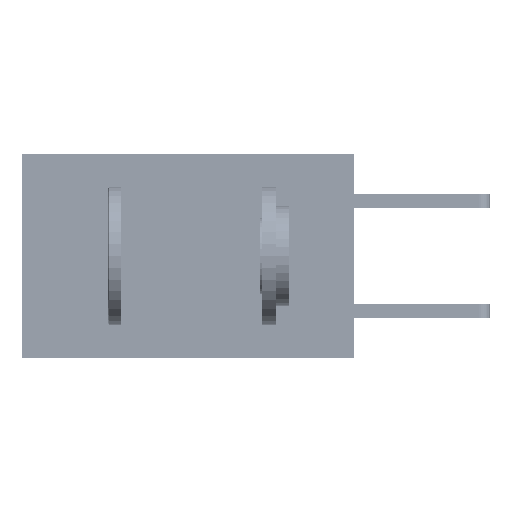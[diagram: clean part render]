
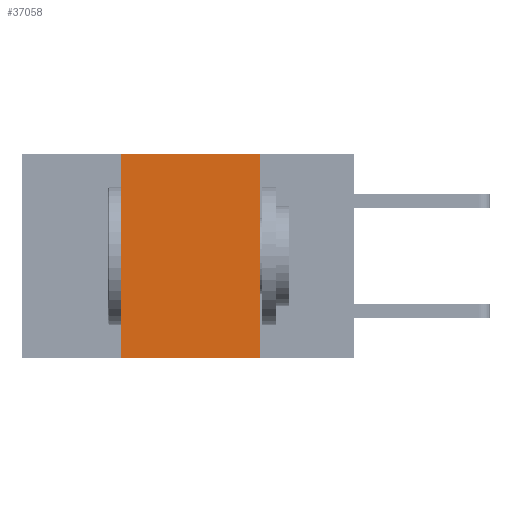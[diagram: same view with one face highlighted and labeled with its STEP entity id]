
A CAD part, left-side view. The second image highlights one B-rep face of the part: STEP entity #37058.
In plain terms, the highlighted planar face has unit normal (-1, 0, 0).
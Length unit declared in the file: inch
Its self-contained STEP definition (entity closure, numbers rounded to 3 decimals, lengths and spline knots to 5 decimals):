
#285 = EDGE_CURVE ( 'NONE', #36489, #21820, #44807, .T. ) ;
#646 = DIRECTION ( 'NONE',  ( 0., -1., 0. ) ) ;
#5187 = ORIENTED_EDGE ( 'NONE', *, *, #48113, .F. ) ;
#6625 = LINE ( 'NONE', #11080, #50487 ) ;
#7666 = VECTOR ( 'NONE', #37270, 39.37008 ) ;
#9012 = ORIENTED_EDGE ( 'NONE', *, *, #38375, .F. ) ;
#9309 = CARTESIAN_POINT ( 'NONE',  ( 0., 0.6, -0.37 ) ) ;
#9411 = CARTESIAN_POINT ( 'NONE',  ( 0., 0.17, 0. ) ) ;
#9585 = VERTEX_POINT ( 'NONE', #37923 ) ;
#9885 = CARTESIAN_POINT ( 'NONE',  ( 0., 0.17, -0.37 ) ) ;
#10435 = DIRECTION ( 'NONE',  ( 0., 0., -1. ) ) ;
#10575 = DIRECTION ( 'NONE',  ( 0., 0., 1. ) ) ;
#11080 = CARTESIAN_POINT ( 'NONE',  ( 0., 0.42, 0. ) ) ;
#11533 = VECTOR ( 'NONE', #646, 39.37008 ) ;
#13605 = DIRECTION ( 'NONE',  ( 1., 0., 0. ) ) ;
#13886 = LINE ( 'NONE', #46690, #35745 ) ;
#21116 = EDGE_CURVE ( 'NONE', #24123, #21820, #49351, .T. ) ;
#21753 = DIRECTION ( 'NONE',  ( 0., -1., 0. ) ) ;
#21820 = VERTEX_POINT ( 'NONE', #9885 ) ;
#24123 = VERTEX_POINT ( 'NONE', #9411 ) ;
#29151 = CARTESIAN_POINT ( 'NONE',  ( 0., 0.17, 0. ) ) ;
#33556 = PLANE ( 'NONE',  #47368 ) ;
#33822 = FACE_OUTER_BOUND ( 'NONE', #51465, .T. ) ;
#35745 = VECTOR ( 'NONE', #21753, 39.37008 ) ;
#36489 = VERTEX_POINT ( 'NONE', #36987 ) ;
#36987 = CARTESIAN_POINT ( 'NONE',  ( 0., 0.42, -0.37 ) ) ;
#37058 = ADVANCED_FACE ( 'NONE', ( #33822 ), #33556, .F. ) ;
#37270 = DIRECTION ( 'NONE',  ( 0., 0., -1. ) ) ;
#37923 = CARTESIAN_POINT ( 'NONE',  ( 0., 0.42, 0. ) ) ;
#38375 = EDGE_CURVE ( 'NONE', #9585, #24123, #13886, .T. ) ;
#38711 = ORIENTED_EDGE ( 'NONE', *, *, #21116, .F. ) ;
#38746 = ORIENTED_EDGE ( 'NONE', *, *, #285, .T. ) ;
#44807 = LINE ( 'NONE', #9309, #11533 ) ;
#46690 = CARTESIAN_POINT ( 'NONE',  ( 0., 0.6, 0. ) ) ;
#47368 = AXIS2_PLACEMENT_3D ( 'NONE', #50355, #13605, #10435 ) ;
#48113 = EDGE_CURVE ( 'NONE', #36489, #9585, #6625, .T. ) ;
#49351 = LINE ( 'NONE', #29151, #7666 ) ;
#50355 = CARTESIAN_POINT ( 'NONE',  ( 0., 0.6, 0. ) ) ;
#50487 = VECTOR ( 'NONE', #10575, 39.37008 ) ;
#51465 = EDGE_LOOP ( 'NONE', ( #38711, #9012, #5187, #38746 ) ) ;
